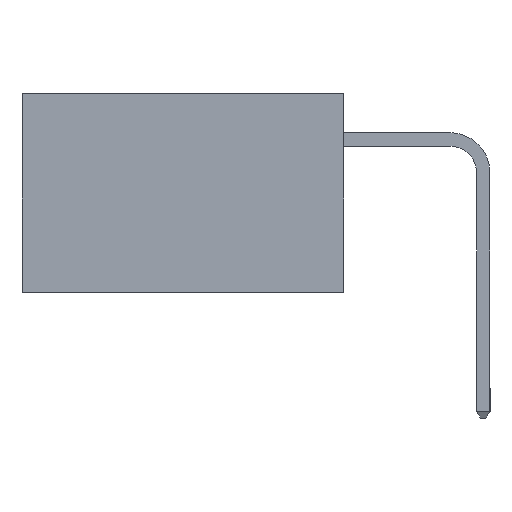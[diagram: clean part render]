
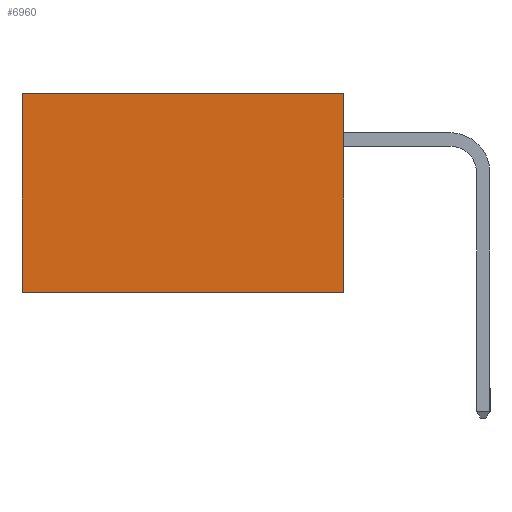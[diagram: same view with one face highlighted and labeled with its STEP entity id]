
A CAD part, left-side view. The second image highlights one B-rep face of the part: STEP entity #6960.
In plain terms, the highlighted planar face has unit normal (-1, 0, 0).
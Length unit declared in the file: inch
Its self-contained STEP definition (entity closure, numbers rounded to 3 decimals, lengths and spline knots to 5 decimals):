
#471 = LINE ( 'NONE', #16895, #7613 ) ;
#1423 = EDGE_CURVE ( 'NONE', #17996, #13500, #3763, .T. ) ;
#1435 = VECTOR ( 'NONE', #11558, 39.37008 ) ;
#1529 = DIRECTION ( 'NONE',  ( 1., 0., 0. ) ) ;
#1531 = DIRECTION ( 'NONE',  ( 0., 0., -1. ) ) ;
#1574 = ORIENTED_EDGE ( 'NONE', *, *, #8559, .F. ) ;
#3639 = VECTOR ( 'NONE', #10040, 39.37008 ) ;
#3763 = LINE ( 'NONE', #12221, #11652 ) ;
#5510 = AXIS2_PLACEMENT_3D ( 'NONE', #7177, #1529, #1531 ) ;
#5566 = EDGE_LOOP ( 'NONE', ( #11517, #9395, #1574, #8291 ) ) ;
#6960 = ADVANCED_FACE ( 'NONE', ( #9814 ), #9439, .F. ) ;
#7177 = CARTESIAN_POINT ( 'NONE',  ( 0.298, 0., 0. ) ) ;
#7613 = VECTOR ( 'NONE', #17060, 39.37008 ) ;
#8291 = ORIENTED_EDGE ( 'NONE', *, *, #1423, .T. ) ;
#8559 = EDGE_CURVE ( 'NONE', #17996, #13078, #9029, .T. ) ;
#8979 = CARTESIAN_POINT ( 'NONE',  ( 0.298, 0.6, -0.37 ) ) ;
#9029 = LINE ( 'NONE', #14352, #1435 ) ;
#9395 = ORIENTED_EDGE ( 'NONE', *, *, #9954, .F. ) ;
#9439 = PLANE ( 'NONE',  #5510 ) ;
#9814 = FACE_OUTER_BOUND ( 'NONE', #5566, .T. ) ;
#9954 = EDGE_CURVE ( 'NONE', #13078, #11546, #471, .T. ) ;
#10040 = DIRECTION ( 'NONE',  ( 0., 0., -1. ) ) ;
#10162 = EDGE_CURVE ( 'NONE', #13500, #11546, #14842, .T. ) ;
#10590 = CARTESIAN_POINT ( 'NONE',  ( 0.298, 0.6, 0. ) ) ;
#11039 = CARTESIAN_POINT ( 'NONE',  ( 0.298, 0., 0. ) ) ;
#11517 = ORIENTED_EDGE ( 'NONE', *, *, #10162, .T. ) ;
#11546 = VERTEX_POINT ( 'NONE', #8979 ) ;
#11558 = DIRECTION ( 'NONE',  ( 0., 0., -1. ) ) ;
#11652 = VECTOR ( 'NONE', #14409, 39.37008 ) ;
#12221 = CARTESIAN_POINT ( 'NONE',  ( 0.298, 0., 0. ) ) ;
#13078 = VERTEX_POINT ( 'NONE', #14953 ) ;
#13500 = VERTEX_POINT ( 'NONE', #17390 ) ;
#14352 = CARTESIAN_POINT ( 'NONE',  ( 0.298, 0., 0. ) ) ;
#14409 = DIRECTION ( 'NONE',  ( 0., 1., 0. ) ) ;
#14842 = LINE ( 'NONE', #10590, #3639 ) ;
#14953 = CARTESIAN_POINT ( 'NONE',  ( 0.298, 0., -0.37 ) ) ;
#16895 = CARTESIAN_POINT ( 'NONE',  ( 0.298, 0., -0.37 ) ) ;
#17060 = DIRECTION ( 'NONE',  ( 0., 1., 0. ) ) ;
#17390 = CARTESIAN_POINT ( 'NONE',  ( 0.298, 0.6, 0. ) ) ;
#17996 = VERTEX_POINT ( 'NONE', #11039 ) ;
